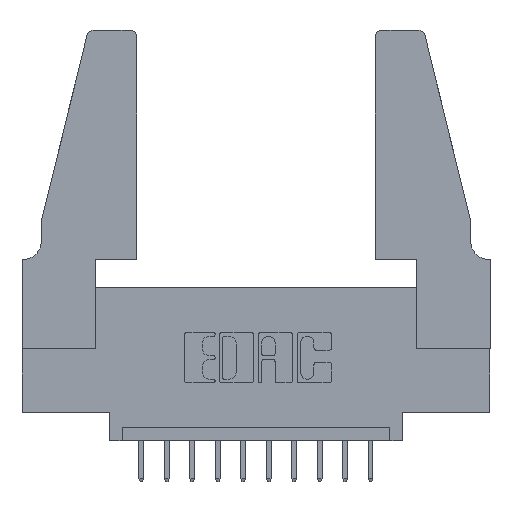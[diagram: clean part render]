
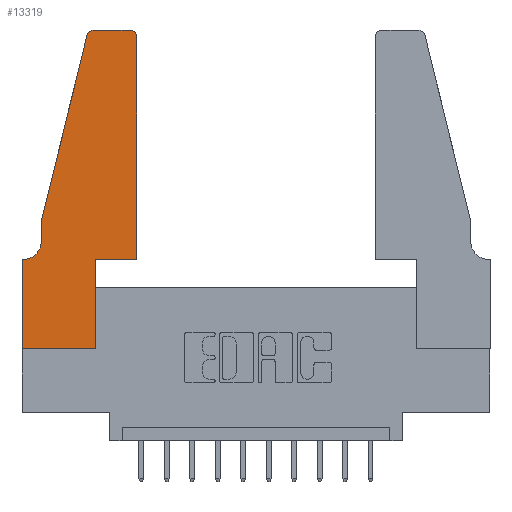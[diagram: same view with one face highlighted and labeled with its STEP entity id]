
A CAD part, top view. The second image highlights one B-rep face of the part: STEP entity #13319.
In plain terms, the highlighted planar face has unit normal (0, 0, 1).
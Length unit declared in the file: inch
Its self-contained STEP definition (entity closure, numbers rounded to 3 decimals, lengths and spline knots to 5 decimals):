
#64 = DIRECTION ( 'NONE',  ( 0., -1., 0. ) ) ;
#171 = ORIENTED_EDGE ( 'NONE', *, *, #10888, .T. ) ;
#208 = ORIENTED_EDGE ( 'NONE', *, *, #13045, .T. ) ;
#439 = PLANE ( 'NONE',  #9878 ) ;
#635 = AXIS2_PLACEMENT_3D ( 'NONE', #9639, #8383, #4001 ) ;
#829 = AXIS2_PLACEMENT_3D ( 'NONE', #13786, #9302, #13881 ) ;
#838 = FACE_OUTER_BOUND ( 'NONE', #7641, .T. ) ;
#842 = CARTESIAN_POINT ( 'NONE',  ( 0.284, 1.25, 0.37 ) ) ;
#859 = VERTEX_POINT ( 'NONE', #6352 ) ;
#1003 = LINE ( 'NONE', #11155, #2222 ) ;
#1134 = DIRECTION ( 'NONE',  ( -1., 0., 0. ) ) ;
#2222 = VECTOR ( 'NONE', #1134, 39.37008 ) ;
#2291 = EDGE_CURVE ( 'NONE', #8539, #9502, #7206, .T. ) ;
#2715 = DIRECTION ( 'NONE',  ( -1., 0., 0. ) ) ;
#2797 = DIRECTION ( 'NONE',  ( 1., 0., 0. ) ) ;
#2982 = VECTOR ( 'NONE', #3978, 39.37008 ) ;
#3160 = ORIENTED_EDGE ( 'NONE', *, *, #13675, .T. ) ;
#3171 = EDGE_CURVE ( 'NONE', #14047, #11465, #6335, .T. ) ;
#3571 = ORIENTED_EDGE ( 'NONE', *, *, #3668, .T. ) ;
#3668 = EDGE_CURVE ( 'NONE', #11808, #10419, #8892, .T. ) ;
#3885 = AXIS2_PLACEMENT_3D ( 'NONE', #4171, #6504, #11875 ) ;
#3978 = DIRECTION ( 'NONE',  ( 1., 0., 0. ) ) ;
#4001 = DIRECTION ( 'NONE',  ( 1., 0., 0. ) ) ;
#4040 = ORIENTED_EDGE ( 'NONE', *, *, #7419, .T. ) ;
#4073 = DIRECTION ( 'NONE',  ( 0., -1., 0. ) ) ;
#4171 = CARTESIAN_POINT ( 'NONE',  ( 0.0055, 0.42, 0.37 ) ) ;
#4277 = CARTESIAN_POINT ( 'NONE',  ( 0., 0., 0.37 ) ) ;
#4307 = DIRECTION ( 'NONE',  ( -0.239, -0.971, 0. ) ) ;
#4366 = ORIENTED_EDGE ( 'NONE', *, *, #12180, .T. ) ;
#4497 = LINE ( 'NONE', #12917, #7254 ) ;
#4840 = LINE ( 'NONE', #6218, #8976 ) ;
#4966 = DIRECTION ( 'NONE',  ( 0., 0., 1. ) ) ;
#4993 = VERTEX_POINT ( 'NONE', #4277 ) ;
#5574 = ORIENTED_EDGE ( 'NONE', *, *, #3171, .T. ) ;
#6215 = VERTEX_POINT ( 'NONE', #6708 ) ;
#6218 = CARTESIAN_POINT ( 'NONE',  ( 0., 0., 0.37 ) ) ;
#6335 = CIRCLE ( 'NONE', #829, 0.03 ) ;
#6352 = CARTESIAN_POINT ( 'NONE',  ( 0.2865, 0., 0.37 ) ) ;
#6504 = DIRECTION ( 'NONE',  ( 0., 0., -1. ) ) ;
#6708 = CARTESIAN_POINT ( 'NONE',  ( 0., 0.35, 0.37 ) ) ;
#6875 = LINE ( 'NONE', #7851, #13903 ) ;
#6879 = EDGE_CURVE ( 'NONE', #10361, #11405, #10894, .T. ) ;
#7023 = CARTESIAN_POINT ( 'NONE',  ( 0.4505, 1.22, 0.37 ) ) ;
#7041 = DIRECTION ( 'NONE',  ( 0., 1., 0. ) ) ;
#7206 = CIRCLE ( 'NONE', #635, 0.03 ) ;
#7254 = VECTOR ( 'NONE', #4073, 39.37008 ) ;
#7331 = ORIENTED_EDGE ( 'NONE', *, *, #11636, .T. ) ;
#7419 = EDGE_CURVE ( 'NONE', #859, #10361, #7621, .T. ) ;
#7621 = LINE ( 'NONE', #9083, #10038 ) ;
#7641 = EDGE_LOOP ( 'NONE', ( #171, #12123, #12025, #4366, #3571, #3160, #208, #11070, #4040, #7706, #7331, #5574 ) ) ;
#7706 = ORIENTED_EDGE ( 'NONE', *, *, #6879, .T. ) ;
#7846 = EDGE_CURVE ( 'NONE', #4993, #859, #4840, .T. ) ;
#7851 = CARTESIAN_POINT ( 'NONE',  ( 0., 0., 0.37 ) ) ;
#8383 = DIRECTION ( 'NONE',  ( 0., 0., 1. ) ) ;
#8405 = CARTESIAN_POINT ( 'NONE',  ( 0.2865, 0.35, 0.37 ) ) ;
#8539 = VERTEX_POINT ( 'NONE', #842 ) ;
#8892 = CIRCLE ( 'NONE', #3885, 0.07 ) ;
#8976 = VECTOR ( 'NONE', #12383, 39.37008 ) ;
#9000 = CARTESIAN_POINT ( 'NONE',  ( 0.0755, 0.42, 0.37 ) ) ;
#9083 = CARTESIAN_POINT ( 'NONE',  ( 0.2865, 0.35, 0.37 ) ) ;
#9302 = DIRECTION ( 'NONE',  ( 0., 0., 1. ) ) ;
#9502 = VERTEX_POINT ( 'NONE', #13673 ) ;
#9639 = CARTESIAN_POINT ( 'NONE',  ( 0.284, 1.22, 0.37 ) ) ;
#9679 = LINE ( 'NONE', #12560, #13949 ) ;
#9878 = AXIS2_PLACEMENT_3D ( 'NONE', #12694, #4966, #2797 ) ;
#9890 = CARTESIAN_POINT ( 'NONE',  ( 0.0055, 0.35, 0.37 ) ) ;
#10038 = VECTOR ( 'NONE', #7041, 39.37008 ) ;
#10361 = VERTEX_POINT ( 'NONE', #8405 ) ;
#10419 = VERTEX_POINT ( 'NONE', #9890 ) ;
#10725 = DIRECTION ( 'NONE',  ( 0., 1., 0. ) ) ;
#10888 = EDGE_CURVE ( 'NONE', #11465, #8539, #9679, .T. ) ;
#10894 = LINE ( 'NONE', #13158, #2982 ) ;
#10971 = CARTESIAN_POINT ( 'NONE',  ( 0.0755, 0.5, 0.37 ) ) ;
#11070 = ORIENTED_EDGE ( 'NONE', *, *, #7846, .T. ) ;
#11155 = CARTESIAN_POINT ( 'NONE',  ( 0.0755, 0.35, 0.37 ) ) ;
#11313 = VECTOR ( 'NONE', #4307, 39.37008 ) ;
#11405 = VERTEX_POINT ( 'NONE', #13785 ) ;
#11465 = VERTEX_POINT ( 'NONE', #12698 ) ;
#11636 = EDGE_CURVE ( 'NONE', #11405, #14047, #13088, .T. ) ;
#11808 = VERTEX_POINT ( 'NONE', #9000 ) ;
#11875 = DIRECTION ( 'NONE',  ( -1., 0., 0. ) ) ;
#12025 = ORIENTED_EDGE ( 'NONE', *, *, #13776, .T. ) ;
#12123 = ORIENTED_EDGE ( 'NONE', *, *, #2291, .T. ) ;
#12180 = EDGE_CURVE ( 'NONE', #12754, #11808, #4497, .T. ) ;
#12347 = LINE ( 'NONE', #10971, #11313 ) ;
#12383 = DIRECTION ( 'NONE',  ( 1., 0., 0. ) ) ;
#12560 = CARTESIAN_POINT ( 'NONE',  ( 0.2605, 1.25, 0.37 ) ) ;
#12694 = CARTESIAN_POINT ( 'NONE',  ( 0., 0.35, 0.37 ) ) ;
#12698 = CARTESIAN_POINT ( 'NONE',  ( 0.4205, 1.25, 0.37 ) ) ;
#12754 = VERTEX_POINT ( 'NONE', #12806 ) ;
#12806 = CARTESIAN_POINT ( 'NONE',  ( 0.0755, 0.5, 0.37 ) ) ;
#12917 = CARTESIAN_POINT ( 'NONE',  ( 0.0755, 0.5, 0.37 ) ) ;
#12933 = VECTOR ( 'NONE', #10725, 39.37008 ) ;
#13045 = EDGE_CURVE ( 'NONE', #6215, #4993, #6875, .T. ) ;
#13088 = LINE ( 'NONE', #13972, #12933 ) ;
#13158 = CARTESIAN_POINT ( 'NONE',  ( 0.4505, 0.35, 0.37 ) ) ;
#13319 = ADVANCED_FACE ( 'NONE', ( #838 ), #439, .T. ) ;
#13673 = CARTESIAN_POINT ( 'NONE',  ( 0.25487, 1.22718, 0.37 ) ) ;
#13675 = EDGE_CURVE ( 'NONE', #10419, #6215, #1003, .T. ) ;
#13776 = EDGE_CURVE ( 'NONE', #9502, #12754, #12347, .T. ) ;
#13785 = CARTESIAN_POINT ( 'NONE',  ( 0.4505, 0.35, 0.37 ) ) ;
#13786 = CARTESIAN_POINT ( 'NONE',  ( 0.4205, 1.22, 0.37 ) ) ;
#13881 = DIRECTION ( 'NONE',  ( 1., 0., 0. ) ) ;
#13903 = VECTOR ( 'NONE', #64, 39.37008 ) ;
#13949 = VECTOR ( 'NONE', #2715, 39.37008 ) ;
#13972 = CARTESIAN_POINT ( 'NONE',  ( 0.4505, 0.35, 0.37 ) ) ;
#14047 = VERTEX_POINT ( 'NONE', #7023 ) ;
